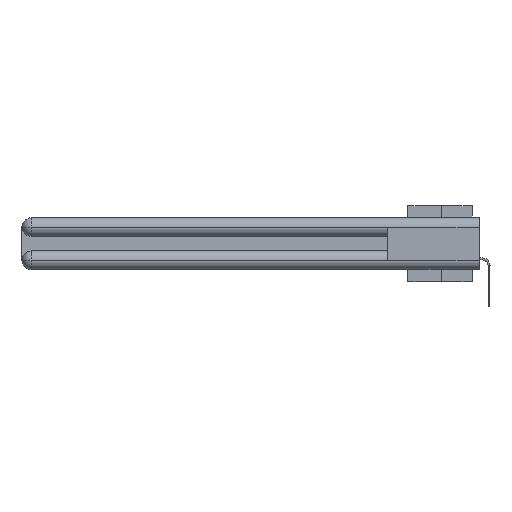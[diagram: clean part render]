
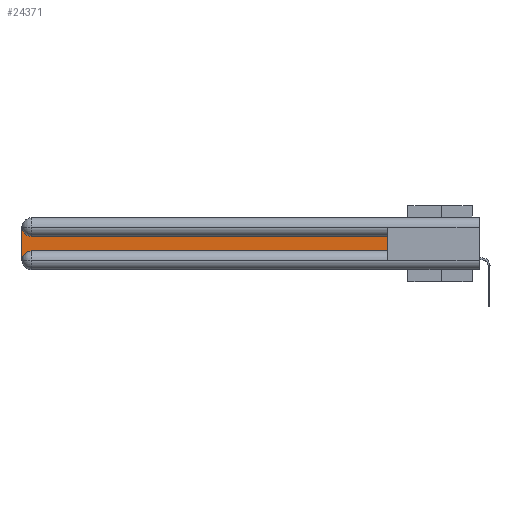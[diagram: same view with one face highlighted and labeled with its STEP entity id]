
A CAD part, left-side view. The second image highlights one B-rep face of the part: STEP entity #24371.
In plain terms, the highlighted planar face has unit normal (-1, 0, 0).
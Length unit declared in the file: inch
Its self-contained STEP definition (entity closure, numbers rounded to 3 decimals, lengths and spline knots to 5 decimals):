
#1710 = DIRECTION ( 'NONE',  ( 0., -1., 0. ) ) ;
#2775 = EDGE_CURVE ( 'NONE', #26033, #23771, #6643, .T. ) ;
#2897 = VECTOR ( 'NONE', #36794, 39.37008 ) ;
#3814 = FACE_OUTER_BOUND ( 'NONE', #10199, .T. ) ;
#4148 = AXIS2_PLACEMENT_3D ( 'NONE', #31720, #13774, #32492 ) ;
#4652 = ORIENTED_EDGE ( 'NONE', *, *, #6268, .T. ) ;
#6268 = EDGE_CURVE ( 'NONE', #28153, #22095, #18688, .T. ) ;
#6564 = VERTEX_POINT ( 'NONE', #10899 ) ;
#6643 = LINE ( 'NONE', #34334, #34785 ) ;
#9460 = EDGE_CURVE ( 'NONE', #6564, #26033, #31980, .T. ) ;
#9729 = DIRECTION ( 'NONE',  ( 1., 0., 0. ) ) ;
#10199 = EDGE_LOOP ( 'NONE', ( #17148, #37661, #29684, #35775, #10253, #4652 ) ) ;
#10253 = ORIENTED_EDGE ( 'NONE', *, *, #36019, .T. ) ;
#10899 = CARTESIAN_POINT ( 'NONE',  ( 0.075, 2.94, -0.1225 ) ) ;
#11072 = EDGE_CURVE ( 'NONE', #22095, #6564, #38334, .T. ) ;
#13774 = DIRECTION ( 'NONE',  ( 1., 0., 0. ) ) ;
#15909 = CARTESIAN_POINT ( 'NONE',  ( 0.075, 0.6, -0.1225 ) ) ;
#16219 = DIRECTION ( 'NONE',  ( 1., 0., 0. ) ) ;
#17144 = CARTESIAN_POINT ( 'NONE',  ( 0.075, 0.6, -0.1225 ) ) ;
#17148 = ORIENTED_EDGE ( 'NONE', *, *, #11072, .T. ) ;
#17693 = EDGE_CURVE ( 'NONE', #23771, #34409, #39210, .T. ) ;
#17756 = CARTESIAN_POINT ( 'NONE',  ( 0.075, 0.6, -0.2175 ) ) ;
#18688 = LINE ( 'NONE', #30465, #2897 ) ;
#20190 = DIRECTION ( 'NONE',  ( 0., 1., 0. ) ) ;
#22095 = VERTEX_POINT ( 'NONE', #15909 ) ;
#22158 = CARTESIAN_POINT ( 'NONE',  ( 0.075, 3., -0.2775 ) ) ;
#22243 = VECTOR ( 'NONE', #20190, 39.37008 ) ;
#23771 = VERTEX_POINT ( 'NONE', #22158 ) ;
#24371 = ADVANCED_FACE ( 'NONE', ( #3814 ), #32283, .F. ) ;
#24890 = VECTOR ( 'NONE', #1710, 39.37008 ) ;
#26033 = VERTEX_POINT ( 'NONE', #32515 ) ;
#28153 = VERTEX_POINT ( 'NONE', #38170 ) ;
#28537 = AXIS2_PLACEMENT_3D ( 'NONE', #34517, #16219, #28619 ) ;
#28619 = DIRECTION ( 'NONE',  ( 0., 0., -1. ) ) ;
#29367 = LINE ( 'NONE', #17756, #24890 ) ;
#29684 = ORIENTED_EDGE ( 'NONE', *, *, #2775, .T. ) ;
#30465 = CARTESIAN_POINT ( 'NONE',  ( 0.075, 0.6, -0.2175 ) ) ;
#31720 = CARTESIAN_POINT ( 'NONE',  ( 0.075, 2.94, -0.2775 ) ) ;
#31980 = CIRCLE ( 'NONE', #32594, 0.06 ) ;
#32283 = PLANE ( 'NONE',  #28537 ) ;
#32492 = DIRECTION ( 'NONE',  ( 0., 0., -1. ) ) ;
#32515 = CARTESIAN_POINT ( 'NONE',  ( 0.075, 3., -0.0625 ) ) ;
#32594 = AXIS2_PLACEMENT_3D ( 'NONE', #37794, #9729, #34531 ) ;
#33055 = CARTESIAN_POINT ( 'NONE',  ( 0.075, 2.94, -0.2175 ) ) ;
#34334 = CARTESIAN_POINT ( 'NONE',  ( 0.075, 3., -0.2175 ) ) ;
#34409 = VERTEX_POINT ( 'NONE', #33055 ) ;
#34517 = CARTESIAN_POINT ( 'NONE',  ( 0.075, 3., -0.1225 ) ) ;
#34531 = DIRECTION ( 'NONE',  ( 0., 0., -1. ) ) ;
#34785 = VECTOR ( 'NONE', #37595, 39.37008 ) ;
#35775 = ORIENTED_EDGE ( 'NONE', *, *, #17693, .T. ) ;
#36019 = EDGE_CURVE ( 'NONE', #34409, #28153, #29367, .T. ) ;
#36794 = DIRECTION ( 'NONE',  ( 0., 0., 1. ) ) ;
#37595 = DIRECTION ( 'NONE',  ( 0., 0., -1. ) ) ;
#37661 = ORIENTED_EDGE ( 'NONE', *, *, #9460, .T. ) ;
#37794 = CARTESIAN_POINT ( 'NONE',  ( 0.075, 2.94, -0.0625 ) ) ;
#38170 = CARTESIAN_POINT ( 'NONE',  ( 0.075, 0.6, -0.2175 ) ) ;
#38334 = LINE ( 'NONE', #17144, #22243 ) ;
#39210 = CIRCLE ( 'NONE', #4148, 0.06 ) ;
